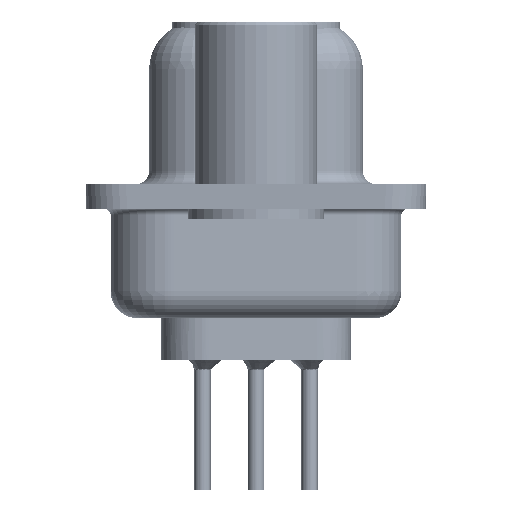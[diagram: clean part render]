
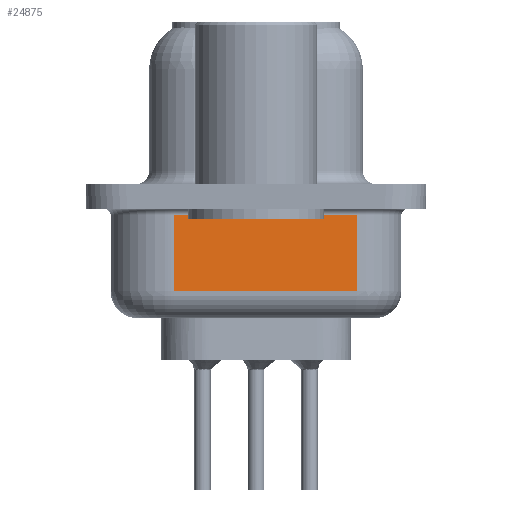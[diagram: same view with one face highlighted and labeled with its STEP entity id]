
A CAD part, left-side view. The second image highlights one B-rep face of the part: STEP entity #24875.
In plain terms, the highlighted planar face has unit normal (-0.985, -0.174, 0).
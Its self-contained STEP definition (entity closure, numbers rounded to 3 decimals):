
#1267 = EDGE_CURVE ( 'NONE', #25544, #5888, #2807, .T. ) ;
#2807 = LINE ( 'NONE', #31394, #43763 ) ;
#3926 = DIRECTION ( 'NONE',  ( 0.174, -0.985, 0. ) ) ;
#5888 = VERTEX_POINT ( 'NONE', #19923 ) ;
#5960 = ORIENTED_EDGE ( 'NONE', *, *, #34480, .T. ) ;
#7267 = PLANE ( 'NONE',  #45862 ) ;
#9125 = CARTESIAN_POINT ( 'NONE',  ( 4.321, -3.722, -0.7 ) ) ;
#9364 = DIRECTION ( 'NONE',  ( -0.174, 0.985, 0. ) ) ;
#13667 = ORIENTED_EDGE ( 'NONE', *, *, #14202, .F. ) ;
#14202 = EDGE_CURVE ( 'NONE', #23745, #5888, #24943, .T. ) ;
#14546 = CARTESIAN_POINT ( 'NONE',  ( 3.13, 3.028, -4.5 ) ) ;
#17791 = CARTESIAN_POINT ( 'NONE',  ( 3.13, 3.028, -3.5 ) ) ;
#17942 = FACE_OUTER_BOUND ( 'NONE', #35142, .T. ) ;
#19923 = CARTESIAN_POINT ( 'NONE',  ( 3.13, 3.028, -0.7 ) ) ;
#22058 = DIRECTION ( 'NONE',  ( -0.174, 0.985, 0. ) ) ;
#23745 = VERTEX_POINT ( 'NONE', #27438 ) ;
#24100 = ORIENTED_EDGE ( 'NONE', *, *, #44797, .T. ) ;
#24875 = ADVANCED_FACE ( 'NONE', ( #17942 ), #7267, .F. ) ;
#24943 = LINE ( 'NONE', #28372, #39208 ) ;
#25544 = VERTEX_POINT ( 'NONE', #9125 ) ;
#27438 = CARTESIAN_POINT ( 'NONE',  ( 3.13, 3.028, -3.5 ) ) ;
#28372 = CARTESIAN_POINT ( 'NONE',  ( 3.13, 3.028, -4.5 ) ) ;
#29143 = LINE ( 'NONE', #17791, #41274 ) ;
#31018 = LINE ( 'NONE', #45594, #39461 ) ;
#31394 = CARTESIAN_POINT ( 'NONE',  ( 3.13, 3.028, -0.7 ) ) ;
#32907 = DIRECTION ( 'NONE',  ( 0.985, 0.174, 0. ) ) ;
#34423 = DIRECTION ( 'NONE',  ( 0., 0., 1. ) ) ;
#34480 = EDGE_CURVE ( 'NONE', #23745, #41133, #29143, .T. ) ;
#34667 = CARTESIAN_POINT ( 'NONE',  ( 4.321, -3.722, -3.5 ) ) ;
#35142 = EDGE_LOOP ( 'NONE', ( #13667, #5960, #24100, #43124 ) ) ;
#39208 = VECTOR ( 'NONE', #39745, 1000. ) ;
#39461 = VECTOR ( 'NONE', #34423, 1000. ) ;
#39745 = DIRECTION ( 'NONE',  ( 0., 0., 1. ) ) ;
#41133 = VERTEX_POINT ( 'NONE', #34667 ) ;
#41274 = VECTOR ( 'NONE', #3926, 1000. ) ;
#43124 = ORIENTED_EDGE ( 'NONE', *, *, #1267, .T. ) ;
#43763 = VECTOR ( 'NONE', #9364, 1000. ) ;
#44797 = EDGE_CURVE ( 'NONE', #41133, #25544, #31018, .T. ) ;
#45594 = CARTESIAN_POINT ( 'NONE',  ( 4.321, -3.722, -4.5 ) ) ;
#45862 = AXIS2_PLACEMENT_3D ( 'NONE', #14546, #32907, #22058 ) ;
